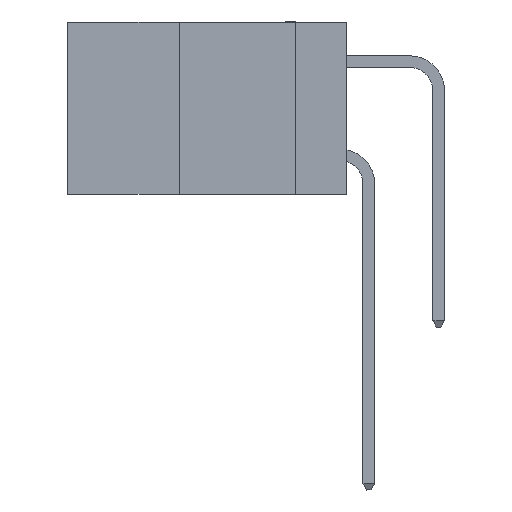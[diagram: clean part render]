
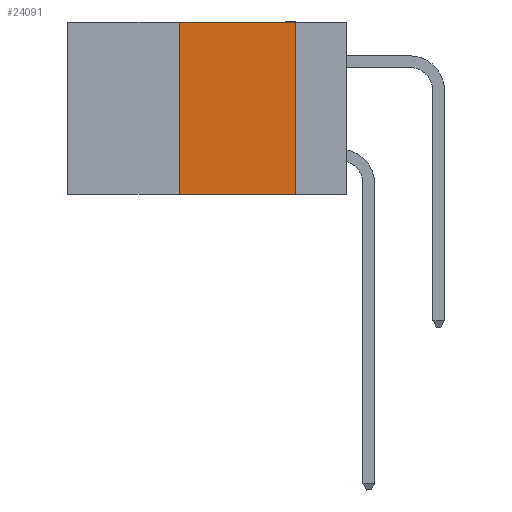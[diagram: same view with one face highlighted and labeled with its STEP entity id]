
A CAD part, left-side view. The second image highlights one B-rep face of the part: STEP entity #24091.
In plain terms, the highlighted planar face has unit normal (-1, 0, 0).
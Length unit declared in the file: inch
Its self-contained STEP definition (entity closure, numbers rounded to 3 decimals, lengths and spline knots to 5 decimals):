
#682 = LINE ( 'NONE', #9906, #17026 ) ;
#1333 = FACE_OUTER_BOUND ( 'NONE', #19286, .T. ) ;
#2260 = VERTEX_POINT ( 'NONE', #6363 ) ;
#4563 = EDGE_CURVE ( 'NONE', #2260, #25148, #15597, .T. ) ;
#5970 = VECTOR ( 'NONE', #21658, 39.37008 ) ;
#6118 = CARTESIAN_POINT ( 'NONE',  ( 0., 0.6, 0. ) ) ;
#6363 = CARTESIAN_POINT ( 'NONE',  ( 0., 0.36, 0. ) ) ;
#6965 = CARTESIAN_POINT ( 'NONE',  ( 0., 0.6, 0. ) ) ;
#9906 = CARTESIAN_POINT ( 'NONE',  ( 0., 0.6, -0.37 ) ) ;
#10412 = VECTOR ( 'NONE', #18248, 39.37008 ) ;
#11257 = VERTEX_POINT ( 'NONE', #30957 ) ;
#13304 = CARTESIAN_POINT ( 'NONE',  ( 0., 0.11, -0.37 ) ) ;
#13327 = EDGE_CURVE ( 'NONE', #25148, #18590, #13827, .T. ) ;
#13679 = VECTOR ( 'NONE', #13694, 39.37008 ) ;
#13694 = DIRECTION ( 'NONE',  ( 0., -1., 0. ) ) ;
#13827 = LINE ( 'NONE', #19177, #5970 ) ;
#15597 = LINE ( 'NONE', #6118, #13679 ) ;
#16754 = ORIENTED_EDGE ( 'NONE', *, *, #4563, .F. ) ;
#17026 = VECTOR ( 'NONE', #30014, 39.37008 ) ;
#18248 = DIRECTION ( 'NONE',  ( 0., 0., 1. ) ) ;
#18590 = VERTEX_POINT ( 'NONE', #13304 ) ;
#19177 = CARTESIAN_POINT ( 'NONE',  ( 0., 0.11, 0. ) ) ;
#19286 = EDGE_LOOP ( 'NONE', ( #22840, #16754, #25152, #21471 ) ) ;
#20442 = CARTESIAN_POINT ( 'NONE',  ( 0., 0.11, 0. ) ) ;
#20925 = EDGE_CURVE ( 'NONE', #11257, #2260, #27875, .T. ) ;
#21471 = ORIENTED_EDGE ( 'NONE', *, *, #28541, .T. ) ;
#21658 = DIRECTION ( 'NONE',  ( 0., 0., -1. ) ) ;
#21867 = PLANE ( 'NONE',  #24654 ) ;
#22840 = ORIENTED_EDGE ( 'NONE', *, *, #13327, .F. ) ;
#23021 = CARTESIAN_POINT ( 'NONE',  ( 0., 0.36, 0. ) ) ;
#24091 = ADVANCED_FACE ( 'NONE', ( #1333 ), #21867, .F. ) ;
#24654 = AXIS2_PLACEMENT_3D ( 'NONE', #6965, #29404, #26434 ) ;
#25148 = VERTEX_POINT ( 'NONE', #20442 ) ;
#25152 = ORIENTED_EDGE ( 'NONE', *, *, #20925, .F. ) ;
#26434 = DIRECTION ( 'NONE',  ( 0., 0., -1. ) ) ;
#27875 = LINE ( 'NONE', #23021, #10412 ) ;
#28541 = EDGE_CURVE ( 'NONE', #11257, #18590, #682, .T. ) ;
#29404 = DIRECTION ( 'NONE',  ( 1., 0., 0. ) ) ;
#30014 = DIRECTION ( 'NONE',  ( 0., -1., 0. ) ) ;
#30957 = CARTESIAN_POINT ( 'NONE',  ( 0., 0.36, -0.37 ) ) ;
